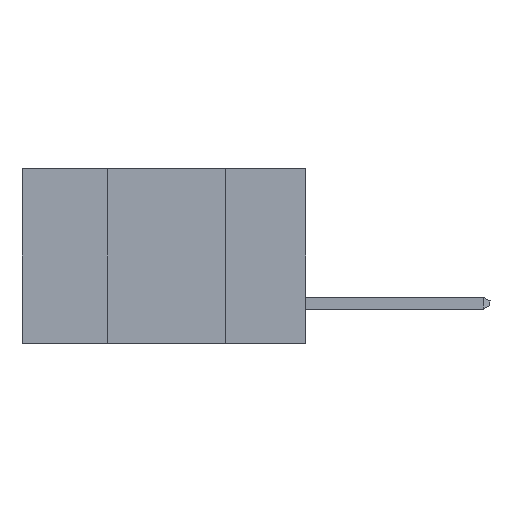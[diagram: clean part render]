
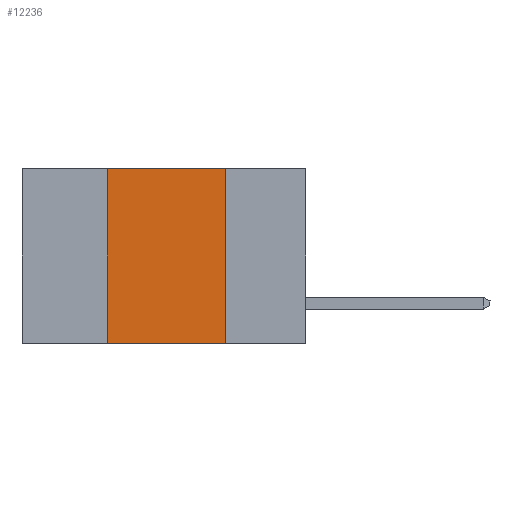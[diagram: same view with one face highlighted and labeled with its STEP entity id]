
A CAD part, left-side view. The second image highlights one B-rep face of the part: STEP entity #12236.
In plain terms, the highlighted planar face has unit normal (-1, 0, 0).
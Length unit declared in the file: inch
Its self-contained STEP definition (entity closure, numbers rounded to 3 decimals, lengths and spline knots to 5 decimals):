
#787 = LINE ( 'NONE', #3768, #5119 ) ;
#867 = ORIENTED_EDGE ( 'NONE', *, *, #2105, .T. ) ;
#944 = CARTESIAN_POINT ( 'NONE',  ( 0., 0.42, -0.37 ) ) ;
#1127 = VECTOR ( 'NONE', #10097, 39.37008 ) ;
#1193 = CARTESIAN_POINT ( 'NONE',  ( 0., 0.6, 0. ) ) ;
#1513 = EDGE_CURVE ( 'NONE', #12136, #5054, #9386, .T. ) ;
#1811 = EDGE_LOOP ( 'NONE', ( #9511, #2629, #12466, #867 ) ) ;
#2105 = EDGE_CURVE ( 'NONE', #12136, #5026, #787, .T. ) ;
#2286 = DIRECTION ( 'NONE',  ( 0., 0., -1. ) ) ;
#2326 = VERTEX_POINT ( 'NONE', #3630 ) ;
#2629 = ORIENTED_EDGE ( 'NONE', *, *, #10026, .F. ) ;
#3201 = PLANE ( 'NONE',  #6585 ) ;
#3336 = VECTOR ( 'NONE', #5151, 39.37008 ) ;
#3630 = CARTESIAN_POINT ( 'NONE',  ( 0., 0.17, 0. ) ) ;
#3709 = CARTESIAN_POINT ( 'NONE',  ( 0., 0.42, 0. ) ) ;
#3768 = CARTESIAN_POINT ( 'NONE',  ( 0., 0.6, -0.37 ) ) ;
#5026 = VERTEX_POINT ( 'NONE', #11316 ) ;
#5054 = VERTEX_POINT ( 'NONE', #3709 ) ;
#5119 = VECTOR ( 'NONE', #7865, 39.37008 ) ;
#5151 = DIRECTION ( 'NONE',  ( 0., 0., -1. ) ) ;
#5230 = CARTESIAN_POINT ( 'NONE',  ( 0., 0.42, -0.37 ) ) ;
#5889 = LINE ( 'NONE', #9055, #1127 ) ;
#6207 = DIRECTION ( 'NONE',  ( 1., 0., 0. ) ) ;
#6216 = EDGE_CURVE ( 'NONE', #2326, #5026, #7958, .T. ) ;
#6281 = DIRECTION ( 'NONE',  ( 0., 0., 1. ) ) ;
#6585 = AXIS2_PLACEMENT_3D ( 'NONE', #1193, #6207, #2286 ) ;
#7865 = DIRECTION ( 'NONE',  ( 0., -1., 0. ) ) ;
#7958 = LINE ( 'NONE', #10091, #3336 ) ;
#9055 = CARTESIAN_POINT ( 'NONE',  ( 0., 0.6, 0. ) ) ;
#9386 = LINE ( 'NONE', #5230, #9824 ) ;
#9511 = ORIENTED_EDGE ( 'NONE', *, *, #6216, .F. ) ;
#9824 = VECTOR ( 'NONE', #6281, 39.37008 ) ;
#10026 = EDGE_CURVE ( 'NONE', #5054, #2326, #5889, .T. ) ;
#10091 = CARTESIAN_POINT ( 'NONE',  ( 0., 0.17, -0.37 ) ) ;
#10094 = FACE_OUTER_BOUND ( 'NONE', #1811, .T. ) ;
#10097 = DIRECTION ( 'NONE',  ( 0., -1., 0. ) ) ;
#11316 = CARTESIAN_POINT ( 'NONE',  ( 0., 0.17, -0.37 ) ) ;
#12136 = VERTEX_POINT ( 'NONE', #944 ) ;
#12236 = ADVANCED_FACE ( 'NONE', ( #10094 ), #3201, .F. ) ;
#12466 = ORIENTED_EDGE ( 'NONE', *, *, #1513, .F. ) ;
